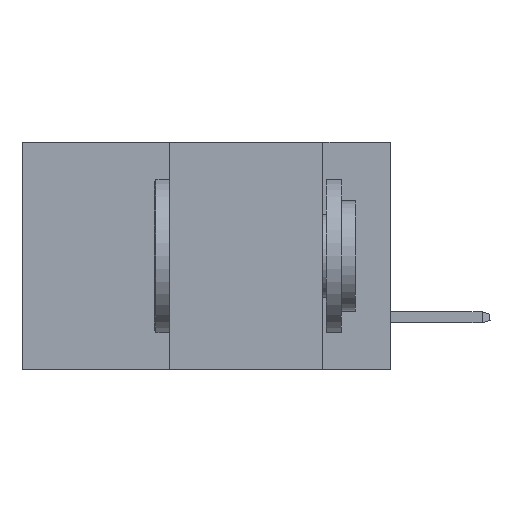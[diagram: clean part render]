
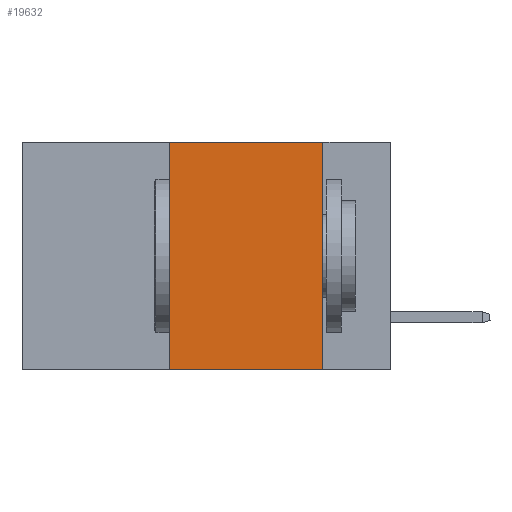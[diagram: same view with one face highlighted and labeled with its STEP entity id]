
A CAD part, left-side view. The second image highlights one B-rep face of the part: STEP entity #19632.
In plain terms, the highlighted planar face has unit normal (-1, 0, 0).
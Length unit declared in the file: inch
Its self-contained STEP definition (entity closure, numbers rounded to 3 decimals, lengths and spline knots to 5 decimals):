
#3078 = DIRECTION ( 'NONE',  ( 0., 0., -1. ) ) ;
#3121 = FACE_OUTER_BOUND ( 'NONE', #17653, .T. ) ;
#3499 = EDGE_CURVE ( 'NONE', #11567, #6597, #33777, .T. ) ;
#3906 = VECTOR ( 'NONE', #28581, 39.37008 ) ;
#4393 = LINE ( 'NONE', #19995, #3906 ) ;
#5913 = EDGE_CURVE ( 'NONE', #6597, #14013, #34740, .T. ) ;
#5994 = VERTEX_POINT ( 'NONE', #25947 ) ;
#6597 = VERTEX_POINT ( 'NONE', #7877 ) ;
#7247 = CARTESIAN_POINT ( 'NONE',  ( 0., 0.6, -0.37 ) ) ;
#7877 = CARTESIAN_POINT ( 'NONE',  ( 0., 0.36, 0. ) ) ;
#8207 = VECTOR ( 'NONE', #27609, 39.37008 ) ;
#11567 = VERTEX_POINT ( 'NONE', #23656 ) ;
#11776 = VECTOR ( 'NONE', #28199, 39.37008 ) ;
#13674 = EDGE_CURVE ( 'NONE', #14013, #5994, #4393, .T. ) ;
#14013 = VERTEX_POINT ( 'NONE', #29856 ) ;
#15110 = CARTESIAN_POINT ( 'NONE',  ( 0., 0.6, 0. ) ) ;
#15986 = DIRECTION ( 'NONE',  ( 0., -1., 0. ) ) ;
#17552 = PLANE ( 'NONE',  #26711 ) ;
#17653 = EDGE_LOOP ( 'NONE', ( #31068, #33285, #33828, #24634 ) ) ;
#17921 = EDGE_CURVE ( 'NONE', #11567, #5994, #33449, .T. ) ;
#19632 = ADVANCED_FACE ( 'NONE', ( #3121 ), #17552, .F. ) ;
#19995 = CARTESIAN_POINT ( 'NONE',  ( 0., 0.11, 0. ) ) ;
#20769 = DIRECTION ( 'NONE',  ( 1., 0., 0. ) ) ;
#22665 = CARTESIAN_POINT ( 'NONE',  ( 0., 0.36, 0. ) ) ;
#22778 = VECTOR ( 'NONE', #15986, 39.37008 ) ;
#23656 = CARTESIAN_POINT ( 'NONE',  ( 0., 0.36, -0.37 ) ) ;
#24634 = ORIENTED_EDGE ( 'NONE', *, *, #17921, .T. ) ;
#25947 = CARTESIAN_POINT ( 'NONE',  ( 0., 0.11, -0.37 ) ) ;
#26711 = AXIS2_PLACEMENT_3D ( 'NONE', #15110, #20769, #3078 ) ;
#27609 = DIRECTION ( 'NONE',  ( 0., -1., 0. ) ) ;
#27893 = CARTESIAN_POINT ( 'NONE',  ( 0., 0.6, 0. ) ) ;
#28199 = DIRECTION ( 'NONE',  ( 0., 0., 1. ) ) ;
#28581 = DIRECTION ( 'NONE',  ( 0., 0., -1. ) ) ;
#29856 = CARTESIAN_POINT ( 'NONE',  ( 0., 0.11, 0. ) ) ;
#31068 = ORIENTED_EDGE ( 'NONE', *, *, #13674, .F. ) ;
#33285 = ORIENTED_EDGE ( 'NONE', *, *, #5913, .F. ) ;
#33449 = LINE ( 'NONE', #7247, #8207 ) ;
#33777 = LINE ( 'NONE', #22665, #11776 ) ;
#33828 = ORIENTED_EDGE ( 'NONE', *, *, #3499, .F. ) ;
#34740 = LINE ( 'NONE', #27893, #22778 ) ;
